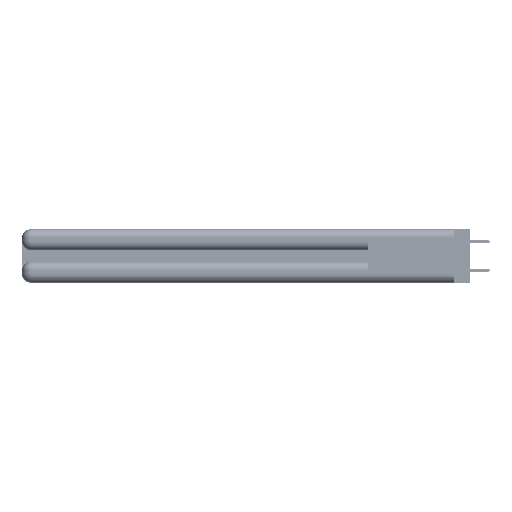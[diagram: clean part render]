
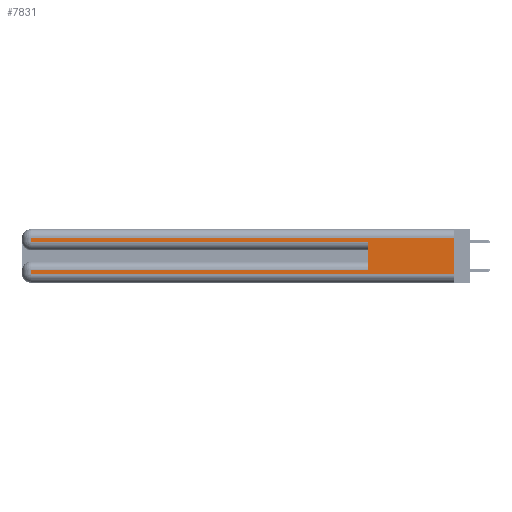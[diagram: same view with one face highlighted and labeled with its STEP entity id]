
A CAD part, left-side view. The second image highlights one B-rep face of the part: STEP entity #7831.
In plain terms, the highlighted planar face has unit normal (-1, 0, 0).
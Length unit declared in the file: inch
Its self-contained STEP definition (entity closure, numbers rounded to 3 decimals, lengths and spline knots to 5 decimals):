
#195 = CARTESIAN_POINT ( 'NONE',  ( 0., 2.94, 0.085 ) ) ;
#251 = CARTESIAN_POINT ( 'NONE',  ( 0., 2.94, 0.31 ) ) ;
#384 = CARTESIAN_POINT ( 'NONE',  ( 0., 0., 0.37 ) ) ;
#829 = ORIENTED_EDGE ( 'NONE', *, *, #9517, .T. ) ;
#1555 = ORIENTED_EDGE ( 'NONE', *, *, #34838, .T. ) ;
#2796 = LINE ( 'NONE', #37514, #46006 ) ;
#3779 = DIRECTION ( 'NONE',  ( 0., 0., -1. ) ) ;
#6055 = VECTOR ( 'NONE', #55386, 39.37008 ) ;
#6418 = ORIENTED_EDGE ( 'NONE', *, *, #47508, .F. ) ;
#7369 = VECTOR ( 'NONE', #34802, 39.37008 ) ;
#7454 = DIRECTION ( 'NONE',  ( 0., 0., -1. ) ) ;
#7708 = LINE ( 'NONE', #7994, #23855 ) ;
#7831 = ADVANCED_FACE ( 'NONE', ( #24421 ), #24581, .F. ) ;
#7994 = CARTESIAN_POINT ( 'NONE',  ( 0., 0.6, 0.145 ) ) ;
#8937 = EDGE_LOOP ( 'NONE', ( #10050, #55594, #829, #1555, #6418, #14689, #13833, #31622 ) ) ;
#9240 = EDGE_CURVE ( 'NONE', #11978, #23323, #31677, .T. ) ;
#9517 = EDGE_CURVE ( 'NONE', #23323, #54278, #54616, .T. ) ;
#10050 = ORIENTED_EDGE ( 'NONE', *, *, #32945, .F. ) ;
#11520 = DIRECTION ( 'NONE',  ( 0., -1., 0. ) ) ;
#11978 = VERTEX_POINT ( 'NONE', #18036 ) ;
#13720 = VECTOR ( 'NONE', #55626, 39.37008 ) ;
#13833 = ORIENTED_EDGE ( 'NONE', *, *, #31205, .T. ) ;
#14007 = VECTOR ( 'NONE', #3779, 39.37008 ) ;
#14437 = EDGE_CURVE ( 'NONE', #44585, #25818, #2796, .T. ) ;
#14689 = ORIENTED_EDGE ( 'NONE', *, *, #14437, .T. ) ;
#15626 = VERTEX_POINT ( 'NONE', #41391 ) ;
#15798 = CARTESIAN_POINT ( 'NONE',  ( 0., 0., 0.31 ) ) ;
#17492 = CARTESIAN_POINT ( 'NONE',  ( 0., 0., 0.06 ) ) ;
#18036 = CARTESIAN_POINT ( 'NONE',  ( 0., 0., 0.31 ) ) ;
#18514 = CARTESIAN_POINT ( 'NONE',  ( 0., 0.6, 0.085 ) ) ;
#20618 = AXIS2_PLACEMENT_3D ( 'NONE', #45777, #23842, #7454 ) ;
#23323 = VERTEX_POINT ( 'NONE', #251 ) ;
#23842 = DIRECTION ( 'NONE',  ( 1., 0., 0. ) ) ;
#23855 = VECTOR ( 'NONE', #37910, 39.37008 ) ;
#24131 = LINE ( 'NONE', #29578, #14007 ) ;
#24421 = FACE_OUTER_BOUND ( 'NONE', #8937, .T. ) ;
#24581 = PLANE ( 'NONE',  #20618 ) ;
#25818 = VERTEX_POINT ( 'NONE', #195 ) ;
#27175 = VERTEX_POINT ( 'NONE', #30767 ) ;
#27936 = LINE ( 'NONE', #36654, #53656 ) ;
#29578 = CARTESIAN_POINT ( 'NONE',  ( 0., 2.94, 0.37 ) ) ;
#30767 = CARTESIAN_POINT ( 'NONE',  ( 0., 2.94, 0.06 ) ) ;
#31205 = EDGE_CURVE ( 'NONE', #25818, #27175, #24131, .T. ) ;
#31622 = ORIENTED_EDGE ( 'NONE', *, *, #38631, .T. ) ;
#31677 = LINE ( 'NONE', #15798, #6055 ) ;
#32945 = EDGE_CURVE ( 'NONE', #11978, #34906, #33516, .T. ) ;
#33516 = LINE ( 'NONE', #384, #45707 ) ;
#33912 = CARTESIAN_POINT ( 'NONE',  ( 0., 0., 0.285 ) ) ;
#34802 = DIRECTION ( 'NONE',  ( 0., 0., -1. ) ) ;
#34838 = EDGE_CURVE ( 'NONE', #54278, #15626, #48184, .T. ) ;
#34906 = VERTEX_POINT ( 'NONE', #17492 ) ;
#36654 = CARTESIAN_POINT ( 'NONE',  ( 0., 0., 0.06 ) ) ;
#37514 = CARTESIAN_POINT ( 'NONE',  ( 0., 0., 0.085 ) ) ;
#37861 = DIRECTION ( 'NONE',  ( 0., 1., 0. ) ) ;
#37910 = DIRECTION ( 'NONE',  ( 0., 0., 1. ) ) ;
#38631 = EDGE_CURVE ( 'NONE', #27175, #34906, #27936, .T. ) ;
#41391 = CARTESIAN_POINT ( 'NONE',  ( 0., 0.6, 0.285 ) ) ;
#44585 = VERTEX_POINT ( 'NONE', #18514 ) ;
#45037 = CARTESIAN_POINT ( 'NONE',  ( 0., 2.94, 0.37 ) ) ;
#45707 = VECTOR ( 'NONE', #50957, 39.37008 ) ;
#45777 = CARTESIAN_POINT ( 'NONE',  ( 0., 0., 0.37 ) ) ;
#46006 = VECTOR ( 'NONE', #37861, 39.37008 ) ;
#46739 = CARTESIAN_POINT ( 'NONE',  ( 0., 2.94, 0.285 ) ) ;
#47508 = EDGE_CURVE ( 'NONE', #44585, #15626, #7708, .T. ) ;
#48184 = LINE ( 'NONE', #33912, #13720 ) ;
#50957 = DIRECTION ( 'NONE',  ( 0., 0., -1. ) ) ;
#53656 = VECTOR ( 'NONE', #11520, 39.37008 ) ;
#54278 = VERTEX_POINT ( 'NONE', #46739 ) ;
#54616 = LINE ( 'NONE', #45037, #7369 ) ;
#55386 = DIRECTION ( 'NONE',  ( 0., 1., 0. ) ) ;
#55594 = ORIENTED_EDGE ( 'NONE', *, *, #9240, .T. ) ;
#55626 = DIRECTION ( 'NONE',  ( 0., -1., 0. ) ) ;
